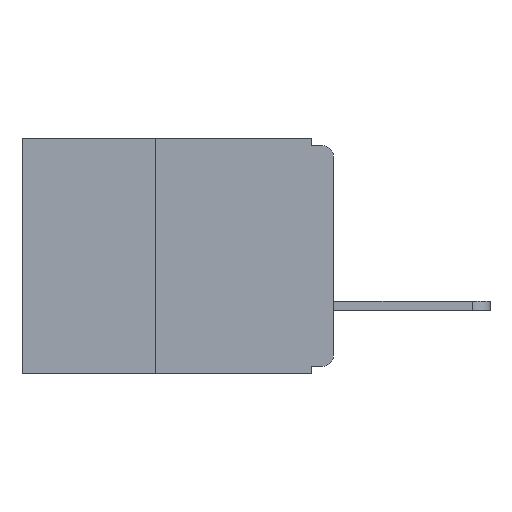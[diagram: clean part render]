
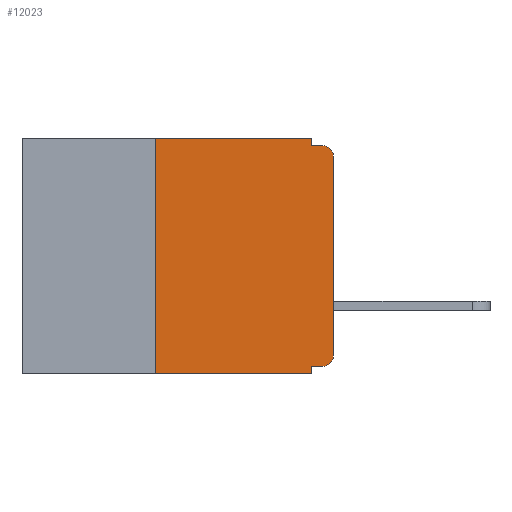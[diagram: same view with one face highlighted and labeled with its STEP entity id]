
A CAD part, left-side view. The second image highlights one B-rep face of the part: STEP entity #12023.
In plain terms, the highlighted planar face has unit normal (-1, 0, 0).
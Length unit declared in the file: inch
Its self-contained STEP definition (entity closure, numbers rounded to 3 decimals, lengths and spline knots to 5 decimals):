
#7 = LINE ( 'NONE', #8451, #330 ) ;
#151 = VECTOR ( 'NONE', #2987, 39.37008 ) ;
#318 = EDGE_CURVE ( 'NONE', #12161, #2857, #6364, .T. ) ;
#330 = VECTOR ( 'NONE', #5195, 39.37008 ) ;
#453 = VECTOR ( 'NONE', #1464, 39.37008 ) ;
#504 = CARTESIAN_POINT ( 'NONE',  ( 0., 0.437, -0.33 ) ) ;
#546 = DIRECTION ( 'NONE',  ( 0., -1., 0. ) ) ;
#763 = VERTEX_POINT ( 'NONE', #7249 ) ;
#821 = VERTEX_POINT ( 'NONE', #3228 ) ;
#955 = DIRECTION ( 'NONE',  ( 0., 0., -1. ) ) ;
#1092 = DIRECTION ( 'NONE',  ( 0., -1., 0. ) ) ;
#1118 = CIRCLE ( 'NONE', #4103, 0.015 ) ;
#1360 = EDGE_CURVE ( 'NONE', #8379, #3647, #10776, .T. ) ;
#1464 = DIRECTION ( 'NONE',  ( 0., -1., 0. ) ) ;
#1844 = LINE ( 'NONE', #4475, #453 ) ;
#1881 = DIRECTION ( 'NONE',  ( 1., 0., 0. ) ) ;
#2097 = ORIENTED_EDGE ( 'NONE', *, *, #13002, .F. ) ;
#2102 = CARTESIAN_POINT ( 'NONE',  ( 0., 0.015, -0.025 ) ) ;
#2263 = VECTOR ( 'NONE', #8999, 39.37008 ) ;
#2550 = ORIENTED_EDGE ( 'NONE', *, *, #8520, .T. ) ;
#2857 = VERTEX_POINT ( 'NONE', #10655 ) ;
#2934 = VERTEX_POINT ( 'NONE', #4628 ) ;
#2987 = DIRECTION ( 'NONE',  ( 0., 1., 0. ) ) ;
#3126 = CARTESIAN_POINT ( 'NONE',  ( 0., 0.031, 0. ) ) ;
#3228 = CARTESIAN_POINT ( 'NONE',  ( 0., 0.015, -0.01 ) ) ;
#3287 = EDGE_CURVE ( 'NONE', #2857, #4850, #7618, .T. ) ;
#3288 = EDGE_CURVE ( 'NONE', #2934, #821, #1118, .T. ) ;
#3504 = CARTESIAN_POINT ( 'NONE',  ( 0., 0.015, -0.305 ) ) ;
#3647 = VERTEX_POINT ( 'NONE', #12857 ) ;
#3848 = VECTOR ( 'NONE', #4741, 39.37008 ) ;
#4103 = AXIS2_PLACEMENT_3D ( 'NONE', #2102, #12218, #12265 ) ;
#4168 = DIRECTION ( 'NONE',  ( 0., 0., -1. ) ) ;
#4313 = DIRECTION ( 'NONE',  ( 0., 0., -1. ) ) ;
#4475 = CARTESIAN_POINT ( 'NONE',  ( 0., 0., -0.01 ) ) ;
#4526 = ORIENTED_EDGE ( 'NONE', *, *, #4553, .F. ) ;
#4553 = EDGE_CURVE ( 'NONE', #11530, #3647, #7, .T. ) ;
#4595 = ORIENTED_EDGE ( 'NONE', *, *, #3288, .T. ) ;
#4627 = ORIENTED_EDGE ( 'NONE', *, *, #8308, .F. ) ;
#4628 = CARTESIAN_POINT ( 'NONE',  ( 0., 0., -0.025 ) ) ;
#4741 = DIRECTION ( 'NONE',  ( 0., 0., 1. ) ) ;
#4850 = VERTEX_POINT ( 'NONE', #5810 ) ;
#5154 = ORIENTED_EDGE ( 'NONE', *, *, #3287, .F. ) ;
#5195 = DIRECTION ( 'NONE',  ( 0., 0., -1. ) ) ;
#5810 = CARTESIAN_POINT ( 'NONE',  ( 0., 0.031, -0.01 ) ) ;
#6095 = CARTESIAN_POINT ( 'NONE',  ( 0., 0.437, 0. ) ) ;
#6126 = AXIS2_PLACEMENT_3D ( 'NONE', #3504, #8437, #4313 ) ;
#6364 = LINE ( 'NONE', #7161, #12379 ) ;
#6556 = LINE ( 'NONE', #6704, #3848 ) ;
#6704 = CARTESIAN_POINT ( 'NONE',  ( 0., 0., 0. ) ) ;
#7161 = CARTESIAN_POINT ( 'NONE',  ( 0., 0.437, 0. ) ) ;
#7249 = CARTESIAN_POINT ( 'NONE',  ( 0., 0.015, -0.32 ) ) ;
#7618 = LINE ( 'NONE', #3126, #11228 ) ;
#7650 = EDGE_CURVE ( 'NONE', #8917, #2934, #6556, .T. ) ;
#7861 = AXIS2_PLACEMENT_3D ( 'NONE', #6095, #1881, #955 ) ;
#7929 = CARTESIAN_POINT ( 'NONE',  ( 0., 0.25, -0.33 ) ) ;
#7996 = CARTESIAN_POINT ( 'NONE',  ( 0., 0.031, -0.32 ) ) ;
#8308 = EDGE_CURVE ( 'NONE', #8379, #12161, #11761, .T. ) ;
#8379 = VERTEX_POINT ( 'NONE', #7929 ) ;
#8392 = CARTESIAN_POINT ( 'NONE',  ( 0., 0., -0.305 ) ) ;
#8437 = DIRECTION ( 'NONE',  ( -1., 0., 0. ) ) ;
#8451 = CARTESIAN_POINT ( 'NONE',  ( 0., 0.031, -0.33 ) ) ;
#8520 = EDGE_CURVE ( 'NONE', #763, #8917, #11633, .T. ) ;
#8917 = VERTEX_POINT ( 'NONE', #8392 ) ;
#8980 = PLANE ( 'NONE',  #7861 ) ;
#8999 = DIRECTION ( 'NONE',  ( 0., 0., 1. ) ) ;
#9045 = VECTOR ( 'NONE', #546, 39.37008 ) ;
#9540 = ORIENTED_EDGE ( 'NONE', *, *, #1360, .T. ) ;
#9799 = LINE ( 'NONE', #10034, #151 ) ;
#10034 = CARTESIAN_POINT ( 'NONE',  ( 0., 0., -0.32 ) ) ;
#10289 = CARTESIAN_POINT ( 'NONE',  ( 0., 0.25, 0. ) ) ;
#10433 = FACE_OUTER_BOUND ( 'NONE', #12061, .T. ) ;
#10655 = CARTESIAN_POINT ( 'NONE',  ( 0., 0.031, 0. ) ) ;
#10776 = LINE ( 'NONE', #504, #9045 ) ;
#11137 = ORIENTED_EDGE ( 'NONE', *, *, #7650, .T. ) ;
#11228 = VECTOR ( 'NONE', #4168, 39.37008 ) ;
#11530 = VERTEX_POINT ( 'NONE', #7996 ) ;
#11633 = CIRCLE ( 'NONE', #6126, 0.015 ) ;
#11761 = LINE ( 'NONE', #11858, #2263 ) ;
#11858 = CARTESIAN_POINT ( 'NONE',  ( 0., 0.25, -0.33 ) ) ;
#11921 = ORIENTED_EDGE ( 'NONE', *, *, #12010, .F. ) ;
#12010 = EDGE_CURVE ( 'NONE', #763, #11530, #9799, .T. ) ;
#12023 = ADVANCED_FACE ( 'NONE', ( #10433 ), #8980, .F. ) ;
#12061 = EDGE_LOOP ( 'NONE', ( #11137, #4595, #2097, #5154, #12168, #4627, #9540, #4526, #11921, #2550 ) ) ;
#12161 = VERTEX_POINT ( 'NONE', #10289 ) ;
#12168 = ORIENTED_EDGE ( 'NONE', *, *, #318, .F. ) ;
#12218 = DIRECTION ( 'NONE',  ( -1., 0., 0. ) ) ;
#12265 = DIRECTION ( 'NONE',  ( 0., 0., -1. ) ) ;
#12379 = VECTOR ( 'NONE', #1092, 39.37008 ) ;
#12857 = CARTESIAN_POINT ( 'NONE',  ( 0., 0.031, -0.33 ) ) ;
#13002 = EDGE_CURVE ( 'NONE', #4850, #821, #1844, .T. ) ;
